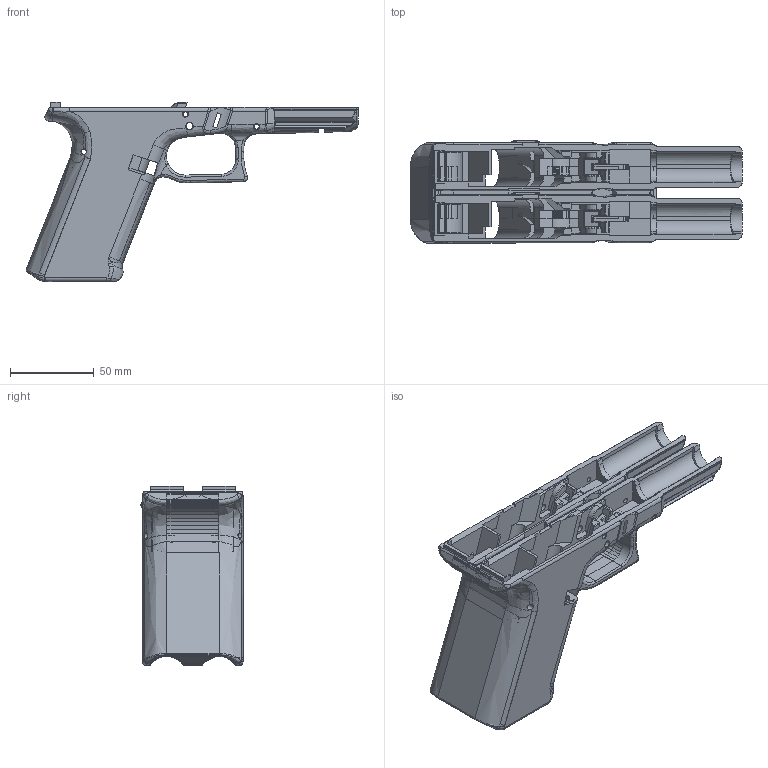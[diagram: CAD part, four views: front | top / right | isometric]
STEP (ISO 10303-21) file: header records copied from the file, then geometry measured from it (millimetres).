
FILE_DESCRIPTION(/* description */ (''),/* implementation_level */ '2;1');
FILE_NAME(/* name */ 'Glocknofsky 17 Beta v4.step',/* time_stamp */ '2022-03-26T10:51:35-04:00',/* author */ (''),/* organization */ (''),/* preprocessor_version */ 'ST-DEVELOPER v18.1',/* originating_system */ 'Autodesk Translation Framework v10.13.0.1454',/* authorisation */ '');
FILE_SCHEMA (('AUTOMOTIVE_DESIGN { 1 0 10303 214 3 1 1 }'));
Products named in the file (2): Glocknofsky 17 Beta v4; Glocknofsky Alpha v1
Assembly tree (1 placements, depth 2):
  Glocknofsky 17 Beta v4
    Glocknofsky Alpha v1
Bounding box: 197.63 x 60.72 x 106.64 mm (x, y, z)
Volume: 217546.8 mm3; surface area: 121505.5 mm2
Topology: 12 solids, 14 shells, 2385 faces, 6717 edges, 4296 vertices
Faces by surface type: plane 1166, bspline 823, cylinder 294, torus 46, sphere 32, cone 24
Full cylindrical faces by diameter (mm): 2 x2, 3 x8, 3.2 x4, 3.5 x1, 4 x4
Entity records: 141993 total; most frequent: CARTESIAN_POINT 86158, ORIENTED_EDGE 13388, DIRECTION 9066, EDGE_CURVE 6694, VERTEX_POINT 4298, LINE 3590, VECTOR 3590, AXIS2_PLACEMENT_3D 2738
